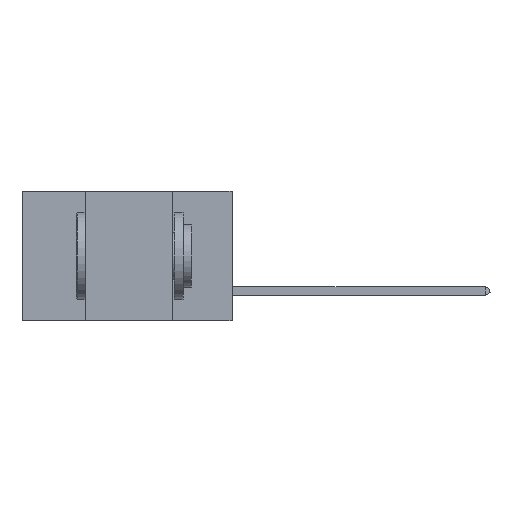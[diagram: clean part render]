
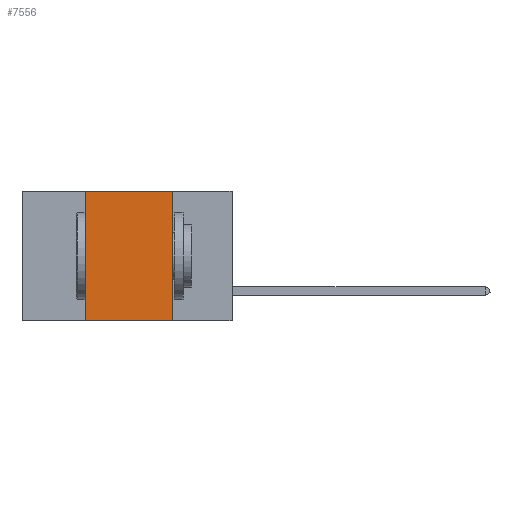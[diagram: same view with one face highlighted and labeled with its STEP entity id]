
A CAD part, left-side view. The second image highlights one B-rep face of the part: STEP entity #7556.
In plain terms, the highlighted planar face has unit normal (-1, 0, 0).
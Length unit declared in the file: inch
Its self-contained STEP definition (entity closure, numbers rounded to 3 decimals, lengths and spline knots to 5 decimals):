
#1017 = DIRECTION ( 'NONE',  ( 1., 0., 0. ) ) ;
#1829 = LINE ( 'NONE', #9067, #11091 ) ;
#2498 = CARTESIAN_POINT ( 'NONE',  ( 0., 0.6, 0. ) ) ;
#3261 = DIRECTION ( 'NONE',  ( 0., 0., 1. ) ) ;
#6804 = ORIENTED_EDGE ( 'NONE', *, *, #34872, .F. ) ;
#7080 = CARTESIAN_POINT ( 'NONE',  ( 0., 0.6, 0. ) ) ;
#7556 = ADVANCED_FACE ( 'NONE', ( #29566 ), #24975, .F. ) ;
#8302 = EDGE_CURVE ( 'NONE', #37092, #14618, #16535, .T. ) ;
#8869 = VECTOR ( 'NONE', #3261, 39.37008 ) ;
#9067 = CARTESIAN_POINT ( 'NONE',  ( 0., 0.6, -0.37 ) ) ;
#9453 = DIRECTION ( 'NONE',  ( 0., -1., 0. ) ) ;
#10509 = VECTOR ( 'NONE', #34665, 39.37008 ) ;
#11073 = VERTEX_POINT ( 'NONE', #21596 ) ;
#11091 = VECTOR ( 'NONE', #9453, 39.37008 ) ;
#12331 = CARTESIAN_POINT ( 'NONE',  ( 0., 0.17, 0. ) ) ;
#12469 = VERTEX_POINT ( 'NONE', #20787 ) ;
#13935 = CARTESIAN_POINT ( 'NONE',  ( 0., 0.17, 0. ) ) ;
#14306 = CARTESIAN_POINT ( 'NONE',  ( 0., 0.42, 0. ) ) ;
#14618 = VERTEX_POINT ( 'NONE', #31318 ) ;
#15106 = EDGE_CURVE ( 'NONE', #12469, #14618, #1829, .T. ) ;
#15764 = DIRECTION ( 'NONE',  ( 0., 0., -1. ) ) ;
#16535 = LINE ( 'NONE', #13935, #10509 ) ;
#19166 = EDGE_CURVE ( 'NONE', #12469, #11073, #38136, .T. ) ;
#20787 = CARTESIAN_POINT ( 'NONE',  ( 0., 0.42, -0.37 ) ) ;
#21596 = CARTESIAN_POINT ( 'NONE',  ( 0., 0.42, 0. ) ) ;
#22112 = ORIENTED_EDGE ( 'NONE', *, *, #8302, .F. ) ;
#22233 = EDGE_LOOP ( 'NONE', ( #22112, #6804, #38410, #30627 ) ) ;
#22854 = LINE ( 'NONE', #2498, #24198 ) ;
#24198 = VECTOR ( 'NONE', #26205, 39.37008 ) ;
#24975 = PLANE ( 'NONE',  #25134 ) ;
#25134 = AXIS2_PLACEMENT_3D ( 'NONE', #7080, #1017, #15764 ) ;
#26205 = DIRECTION ( 'NONE',  ( 0., -1., 0. ) ) ;
#29566 = FACE_OUTER_BOUND ( 'NONE', #22233, .T. ) ;
#30627 = ORIENTED_EDGE ( 'NONE', *, *, #15106, .T. ) ;
#31318 = CARTESIAN_POINT ( 'NONE',  ( 0., 0.17, -0.37 ) ) ;
#34665 = DIRECTION ( 'NONE',  ( 0., 0., -1. ) ) ;
#34872 = EDGE_CURVE ( 'NONE', #11073, #37092, #22854, .T. ) ;
#37092 = VERTEX_POINT ( 'NONE', #12331 ) ;
#38136 = LINE ( 'NONE', #14306, #8869 ) ;
#38410 = ORIENTED_EDGE ( 'NONE', *, *, #19166, .F. ) ;
